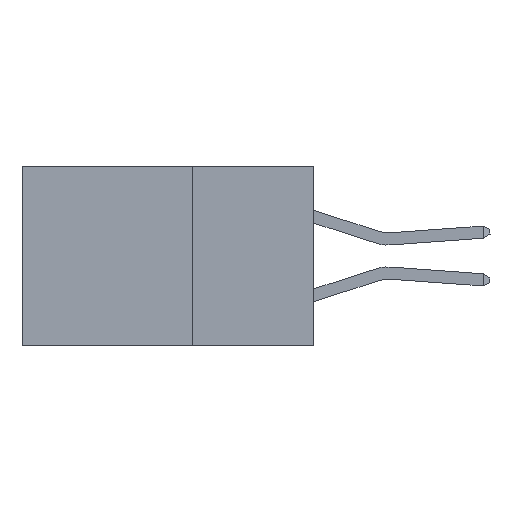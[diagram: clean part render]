
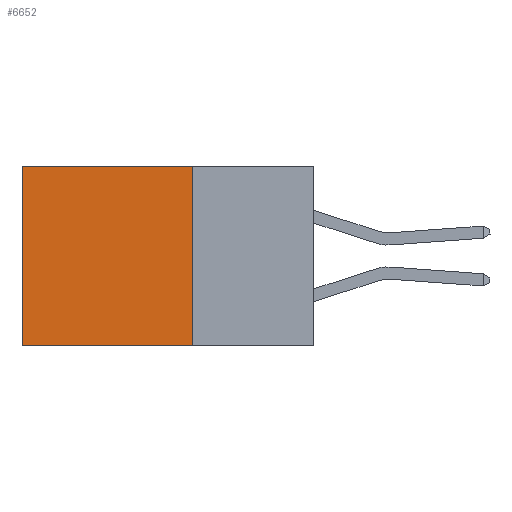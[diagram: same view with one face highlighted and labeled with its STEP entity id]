
A CAD part, left-side view. The second image highlights one B-rep face of the part: STEP entity #6652.
In plain terms, the highlighted planar face has unit normal (-1, 0, 0).
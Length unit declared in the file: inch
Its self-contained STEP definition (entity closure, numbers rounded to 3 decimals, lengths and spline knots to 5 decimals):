
#764 = DIRECTION ( 'NONE',  ( 0., 0., -1. ) ) ;
#862 = VERTEX_POINT ( 'NONE', #10562 ) ;
#3188 = LINE ( 'NONE', #23738, #15987 ) ;
#3657 = CARTESIAN_POINT ( 'NONE',  ( 0.2875, 0.6, 0. ) ) ;
#5082 = EDGE_LOOP ( 'NONE', ( #7470, #7821, #19299, #15138 ) ) ;
#5468 = CARTESIAN_POINT ( 'NONE',  ( 0.2875, 0.25, 0. ) ) ;
#6386 = LINE ( 'NONE', #3657, #24911 ) ;
#6652 = ADVANCED_FACE ( 'NONE', ( #22228 ), #15763, .F. ) ;
#6848 = EDGE_CURVE ( 'NONE', #8010, #22990, #6386, .T. ) ;
#7470 = ORIENTED_EDGE ( 'NONE', *, *, #6848, .T. ) ;
#7821 = ORIENTED_EDGE ( 'NONE', *, *, #21851, .F. ) ;
#8010 = VERTEX_POINT ( 'NONE', #16218 ) ;
#9362 = DIRECTION ( 'NONE',  ( 0., 1., 0. ) ) ;
#9429 = VERTEX_POINT ( 'NONE', #5468 ) ;
#9794 = VECTOR ( 'NONE', #14470, 39.37008 ) ;
#10371 = CARTESIAN_POINT ( 'NONE',  ( 0.2875, 0.25, 0. ) ) ;
#10562 = CARTESIAN_POINT ( 'NONE',  ( 0.2875, 0.25, -0.37 ) ) ;
#12615 = EDGE_CURVE ( 'NONE', #9429, #8010, #16198, .T. ) ;
#13073 = CARTESIAN_POINT ( 'NONE',  ( 0.2875, 0.6, -0.37 ) ) ;
#14470 = DIRECTION ( 'NONE',  ( 0., 1., 0. ) ) ;
#14978 = VECTOR ( 'NONE', #9362, 39.37008 ) ;
#15138 = ORIENTED_EDGE ( 'NONE', *, *, #12615, .T. ) ;
#15763 = PLANE ( 'NONE',  #17249 ) ;
#15987 = VECTOR ( 'NONE', #21494, 39.37008 ) ;
#16198 = LINE ( 'NONE', #10371, #9794 ) ;
#16218 = CARTESIAN_POINT ( 'NONE',  ( 0.2875, 0.6, 0. ) ) ;
#17249 = AXIS2_PLACEMENT_3D ( 'NONE', #21606, #20181, #764 ) ;
#17412 = LINE ( 'NONE', #25052, #14978 ) ;
#18784 = EDGE_CURVE ( 'NONE', #9429, #862, #3188, .T. ) ;
#19299 = ORIENTED_EDGE ( 'NONE', *, *, #18784, .F. ) ;
#20181 = DIRECTION ( 'NONE',  ( 1., 0., 0. ) ) ;
#21494 = DIRECTION ( 'NONE',  ( 0., 0., -1. ) ) ;
#21606 = CARTESIAN_POINT ( 'NONE',  ( 0.2875, 0.25, 0. ) ) ;
#21851 = EDGE_CURVE ( 'NONE', #862, #22990, #17412, .T. ) ;
#21888 = DIRECTION ( 'NONE',  ( 0., 0., -1. ) ) ;
#22228 = FACE_OUTER_BOUND ( 'NONE', #5082, .T. ) ;
#22990 = VERTEX_POINT ( 'NONE', #13073 ) ;
#23738 = CARTESIAN_POINT ( 'NONE',  ( 0.2875, 0.25, 0. ) ) ;
#24911 = VECTOR ( 'NONE', #21888, 39.37008 ) ;
#25052 = CARTESIAN_POINT ( 'NONE',  ( 0.2875, 0.25, -0.37 ) ) ;
